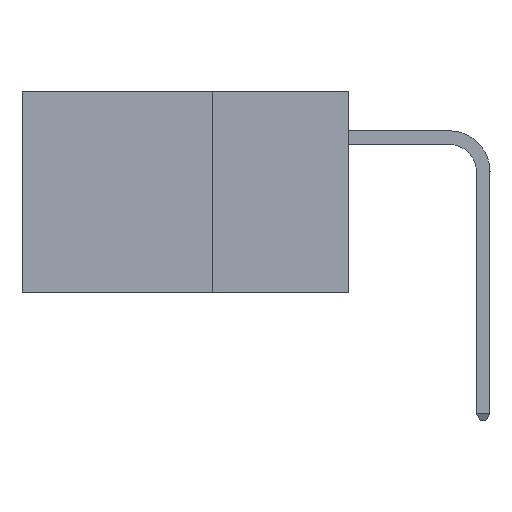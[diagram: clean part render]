
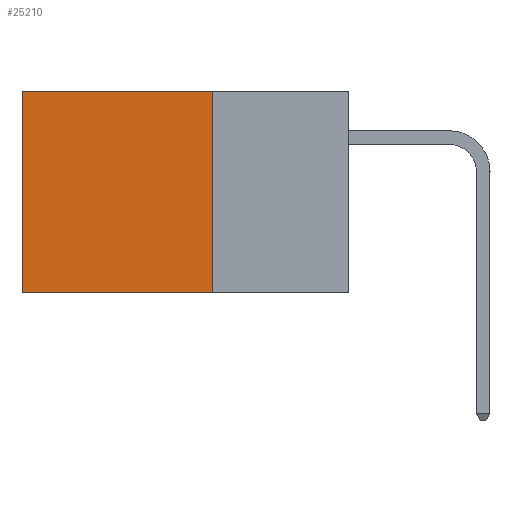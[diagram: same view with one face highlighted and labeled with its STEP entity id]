
A CAD part, left-side view. The second image highlights one B-rep face of the part: STEP entity #25210.
In plain terms, the highlighted planar face has unit normal (-1, 0, 0).
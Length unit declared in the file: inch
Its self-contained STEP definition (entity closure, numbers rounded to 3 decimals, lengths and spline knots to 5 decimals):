
#258 = ORIENTED_EDGE ( 'NONE', *, *, #8679, .T. ) ;
#401 = CARTESIAN_POINT ( 'NONE',  ( 0.2875, 0.6, 0. ) ) ;
#532 = DIRECTION ( 'NONE',  ( 0., 1., 0. ) ) ;
#2174 = VERTEX_POINT ( 'NONE', #6234 ) ;
#2560 = VECTOR ( 'NONE', #14579, 39.37008 ) ;
#4239 = FACE_OUTER_BOUND ( 'NONE', #17770, .T. ) ;
#4429 = EDGE_CURVE ( 'NONE', #2174, #6049, #14279, .T. ) ;
#5149 = EDGE_CURVE ( 'NONE', #24659, #10471, #13287, .T. ) ;
#6049 = VERTEX_POINT ( 'NONE', #19195 ) ;
#6234 = CARTESIAN_POINT ( 'NONE',  ( 0.2875, 0.6, 0. ) ) ;
#7007 = DIRECTION ( 'NONE',  ( 0., 1., 0. ) ) ;
#7046 = LINE ( 'NONE', #22652, #12450 ) ;
#7562 = VECTOR ( 'NONE', #532, 39.37008 ) ;
#8220 = ORIENTED_EDGE ( 'NONE', *, *, #5149, .F. ) ;
#8461 = CARTESIAN_POINT ( 'NONE',  ( 0.2875, 0.25, 0. ) ) ;
#8679 = EDGE_CURVE ( 'NONE', #24659, #2174, #7046, .T. ) ;
#10471 = VERTEX_POINT ( 'NONE', #10708 ) ;
#10529 = DIRECTION ( 'NONE',  ( 0., 0., -1. ) ) ;
#10574 = CARTESIAN_POINT ( 'NONE',  ( 0.2875, 0.25, -0.37 ) ) ;
#10708 = CARTESIAN_POINT ( 'NONE',  ( 0.2875, 0.25, -0.37 ) ) ;
#10880 = CARTESIAN_POINT ( 'NONE',  ( 0.2875, 0.25, 0. ) ) ;
#10889 = ORIENTED_EDGE ( 'NONE', *, *, #16718, .F. ) ;
#12450 = VECTOR ( 'NONE', #7007, 39.37008 ) ;
#12955 = DIRECTION ( 'NONE',  ( 0., 0., -1. ) ) ;
#13242 = CARTESIAN_POINT ( 'NONE',  ( 0.2875, 0.25, 0. ) ) ;
#13287 = LINE ( 'NONE', #8461, #2560 ) ;
#13413 = ORIENTED_EDGE ( 'NONE', *, *, #4429, .T. ) ;
#14279 = LINE ( 'NONE', #401, #18763 ) ;
#14579 = DIRECTION ( 'NONE',  ( 0., 0., -1. ) ) ;
#16718 = EDGE_CURVE ( 'NONE', #10471, #6049, #16915, .T. ) ;
#16763 = PLANE ( 'NONE',  #17271 ) ;
#16915 = LINE ( 'NONE', #10574, #7562 ) ;
#17271 = AXIS2_PLACEMENT_3D ( 'NONE', #10880, #24480, #12955 ) ;
#17770 = EDGE_LOOP ( 'NONE', ( #13413, #10889, #8220, #258 ) ) ;
#18763 = VECTOR ( 'NONE', #10529, 39.37008 ) ;
#19195 = CARTESIAN_POINT ( 'NONE',  ( 0.2875, 0.6, -0.37 ) ) ;
#22652 = CARTESIAN_POINT ( 'NONE',  ( 0.2875, 0.25, 0. ) ) ;
#24480 = DIRECTION ( 'NONE',  ( 1., 0., 0. ) ) ;
#24659 = VERTEX_POINT ( 'NONE', #13242 ) ;
#25210 = ADVANCED_FACE ( 'NONE', ( #4239 ), #16763, .F. ) ;
